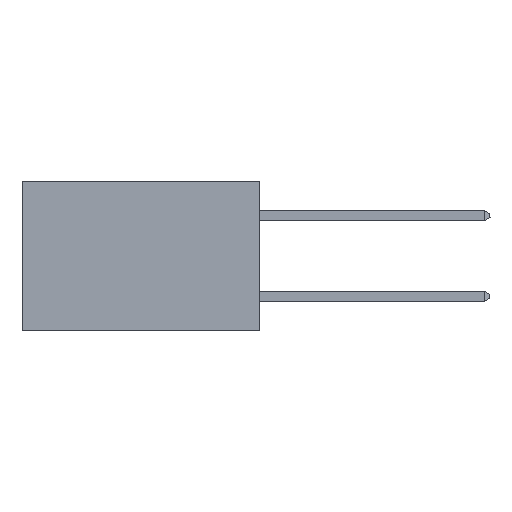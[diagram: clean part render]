
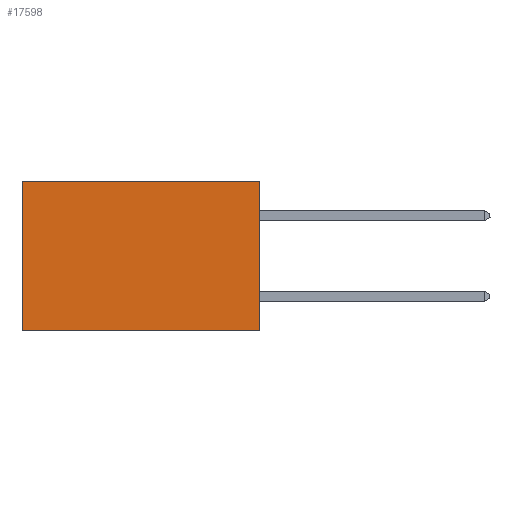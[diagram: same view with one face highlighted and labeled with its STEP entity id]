
A CAD part, left-side view. The second image highlights one B-rep face of the part: STEP entity #17598.
In plain terms, the highlighted planar face has unit normal (-1, 0, 0).
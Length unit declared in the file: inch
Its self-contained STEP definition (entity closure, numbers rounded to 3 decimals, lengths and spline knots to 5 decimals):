
#1194 = VERTEX_POINT ( 'NONE', #10933 ) ;
#2412 = VERTEX_POINT ( 'NONE', #5263 ) ;
#5263 = CARTESIAN_POINT ( 'NONE',  ( 0.277, 0.59, -0.37 ) ) ;
#5745 = VECTOR ( 'NONE', #6907, 39.37008 ) ;
#5830 = CARTESIAN_POINT ( 'NONE',  ( 0.277, 0., 0. ) ) ;
#6088 = VECTOR ( 'NONE', #11915, 39.37008 ) ;
#6708 = CARTESIAN_POINT ( 'NONE',  ( 0.277, 0., -0.37 ) ) ;
#6907 = DIRECTION ( 'NONE',  ( 0., 0., -1. ) ) ;
#7256 = VECTOR ( 'NONE', #7826, 39.37008 ) ;
#7329 = LINE ( 'NONE', #19925, #6088 ) ;
#7826 = DIRECTION ( 'NONE',  ( 0., 1., 0. ) ) ;
#8010 = DIRECTION ( 'NONE',  ( 0., 0., -1. ) ) ;
#9558 = FACE_OUTER_BOUND ( 'NONE', #10872, .T. ) ;
#9955 = EDGE_CURVE ( 'NONE', #12025, #2412, #7329, .T. ) ;
#9995 = CARTESIAN_POINT ( 'NONE',  ( 0.277, 0., -0.37 ) ) ;
#10725 = PLANE ( 'NONE',  #19950 ) ;
#10872 = EDGE_LOOP ( 'NONE', ( #23007, #11720, #22242, #16722 ) ) ;
#10933 = CARTESIAN_POINT ( 'NONE',  ( 0.277, 0., 0. ) ) ;
#11249 = EDGE_CURVE ( 'NONE', #1194, #11767, #17887, .T. ) ;
#11720 = ORIENTED_EDGE ( 'NONE', *, *, #9955, .F. ) ;
#11767 = VERTEX_POINT ( 'NONE', #24857 ) ;
#11869 = VECTOR ( 'NONE', #8010, 39.37008 ) ;
#11915 = DIRECTION ( 'NONE',  ( 0., 1., 0. ) ) ;
#12025 = VERTEX_POINT ( 'NONE', #9995 ) ;
#12482 = LINE ( 'NONE', #23780, #11869 ) ;
#12717 = DIRECTION ( 'NONE',  ( 0., 0., -1. ) ) ;
#12835 = CARTESIAN_POINT ( 'NONE',  ( 0.277, 0., -0.37 ) ) ;
#12962 = EDGE_CURVE ( 'NONE', #1194, #12025, #21616, .T. ) ;
#15439 = EDGE_CURVE ( 'NONE', #11767, #2412, #12482, .T. ) ;
#16722 = ORIENTED_EDGE ( 'NONE', *, *, #11249, .T. ) ;
#17598 = ADVANCED_FACE ( 'NONE', ( #9558 ), #10725, .F. ) ;
#17887 = LINE ( 'NONE', #5830, #7256 ) ;
#19925 = CARTESIAN_POINT ( 'NONE',  ( 0.277, 0., -0.37 ) ) ;
#19950 = AXIS2_PLACEMENT_3D ( 'NONE', #6708, #24418, #12717 ) ;
#21616 = LINE ( 'NONE', #12835, #5745 ) ;
#22242 = ORIENTED_EDGE ( 'NONE', *, *, #12962, .F. ) ;
#23007 = ORIENTED_EDGE ( 'NONE', *, *, #15439, .T. ) ;
#23780 = CARTESIAN_POINT ( 'NONE',  ( 0.277, 0.59, -0.37 ) ) ;
#24418 = DIRECTION ( 'NONE',  ( 1., 0., 0. ) ) ;
#24857 = CARTESIAN_POINT ( 'NONE',  ( 0.277, 0.59, 0. ) ) ;
